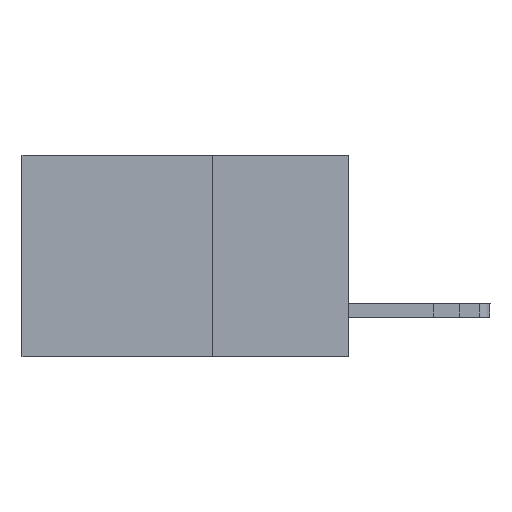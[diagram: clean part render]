
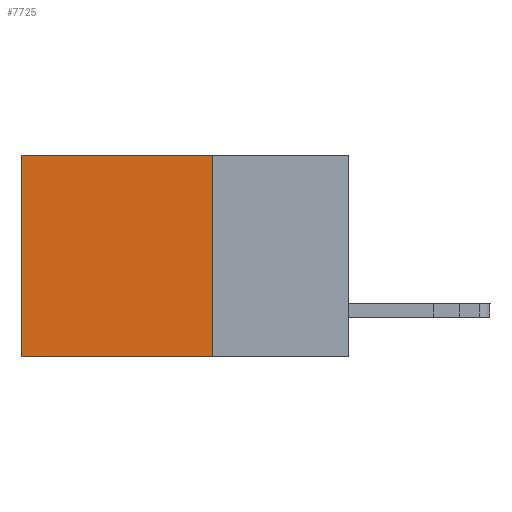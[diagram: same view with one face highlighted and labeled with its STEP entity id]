
A CAD part, left-side view. The second image highlights one B-rep face of the part: STEP entity #7725.
In plain terms, the highlighted planar face has unit normal (-1, 0, 0).
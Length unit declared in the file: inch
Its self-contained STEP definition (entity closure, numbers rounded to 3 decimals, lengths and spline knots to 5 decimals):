
#879 = CARTESIAN_POINT ( 'NONE',  ( 0.2615, 0.25, -0.37 ) ) ;
#1401 = CARTESIAN_POINT ( 'NONE',  ( 0.2615, 0.6, -0.37 ) ) ;
#2092 = ORIENTED_EDGE ( 'NONE', *, *, #11417, .T. ) ;
#3208 = VECTOR ( 'NONE', #5781, 39.37008 ) ;
#3509 = CARTESIAN_POINT ( 'NONE',  ( 0.2615, 0.6, 0. ) ) ;
#3632 = LINE ( 'NONE', #6000, #3208 ) ;
#3795 = EDGE_CURVE ( 'NONE', #16194, #6040, #4995, .T. ) ;
#4157 = ORIENTED_EDGE ( 'NONE', *, *, #10580, .T. ) ;
#4995 = LINE ( 'NONE', #8740, #7982 ) ;
#5730 = ORIENTED_EDGE ( 'NONE', *, *, #6934, .F. ) ;
#5781 = DIRECTION ( 'NONE',  ( 0., 1., 0. ) ) ;
#5789 = LINE ( 'NONE', #14177, #11771 ) ;
#6000 = CARTESIAN_POINT ( 'NONE',  ( 0.2615, 0.25, -0.37 ) ) ;
#6014 = PLANE ( 'NONE',  #6253 ) ;
#6040 = VERTEX_POINT ( 'NONE', #879 ) ;
#6210 = VERTEX_POINT ( 'NONE', #3509 ) ;
#6253 = AXIS2_PLACEMENT_3D ( 'NONE', #12221, #9264, #9048 ) ;
#6854 = DIRECTION ( 'NONE',  ( 0., 0., -1. ) ) ;
#6934 = EDGE_CURVE ( 'NONE', #6040, #8770, #3632, .T. ) ;
#7725 = ADVANCED_FACE ( 'NONE', ( #9946 ), #6014, .F. ) ;
#7982 = VECTOR ( 'NONE', #6854, 39.37008 ) ;
#8430 = VECTOR ( 'NONE', #15103, 39.37008 ) ;
#8718 = EDGE_LOOP ( 'NONE', ( #4157, #5730, #12269, #2092 ) ) ;
#8740 = CARTESIAN_POINT ( 'NONE',  ( 0.2615, 0.25, -0.37 ) ) ;
#8770 = VERTEX_POINT ( 'NONE', #1401 ) ;
#9048 = DIRECTION ( 'NONE',  ( 0., 0., -1. ) ) ;
#9264 = DIRECTION ( 'NONE',  ( 1., 0., 0. ) ) ;
#9946 = FACE_OUTER_BOUND ( 'NONE', #8718, .T. ) ;
#10580 = EDGE_CURVE ( 'NONE', #6210, #8770, #12160, .T. ) ;
#11417 = EDGE_CURVE ( 'NONE', #16194, #6210, #5789, .T. ) ;
#11771 = VECTOR ( 'NONE', #12948, 39.37008 ) ;
#12155 = CARTESIAN_POINT ( 'NONE',  ( 0.2615, 0.25, 0. ) ) ;
#12160 = LINE ( 'NONE', #12704, #8430 ) ;
#12221 = CARTESIAN_POINT ( 'NONE',  ( 0.2615, 0.25, -0.37 ) ) ;
#12269 = ORIENTED_EDGE ( 'NONE', *, *, #3795, .F. ) ;
#12704 = CARTESIAN_POINT ( 'NONE',  ( 0.2615, 0.6, -0.37 ) ) ;
#12948 = DIRECTION ( 'NONE',  ( 0., 1., 0. ) ) ;
#14177 = CARTESIAN_POINT ( 'NONE',  ( 0.2615, 0.25, 0. ) ) ;
#15103 = DIRECTION ( 'NONE',  ( 0., 0., -1. ) ) ;
#16194 = VERTEX_POINT ( 'NONE', #12155 ) ;
